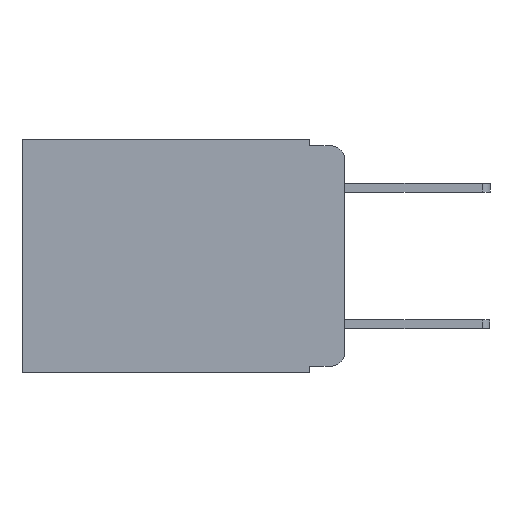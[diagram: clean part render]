
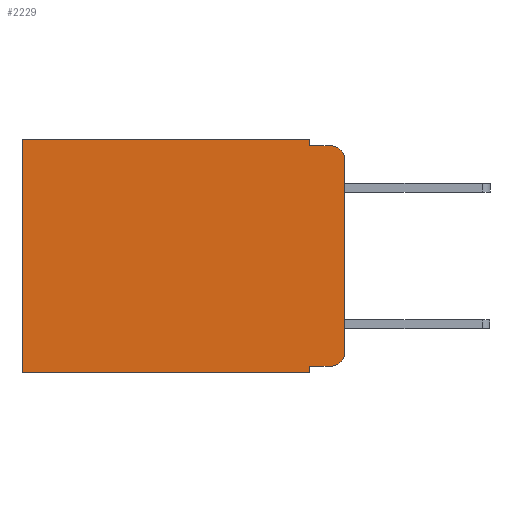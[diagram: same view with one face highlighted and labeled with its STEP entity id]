
A CAD part, left-side view. The second image highlights one B-rep face of the part: STEP entity #2229.
In plain terms, the highlighted planar face has unit normal (-1, 0, 0).
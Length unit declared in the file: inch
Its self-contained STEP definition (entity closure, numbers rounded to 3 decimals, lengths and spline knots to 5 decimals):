
#175 = DIRECTION ( 'NONE',  ( 0., 0., -1. ) ) ;
#256 = LINE ( 'NONE', #12003, #15905 ) ;
#1143 = CARTESIAN_POINT ( 'NONE',  ( 0.298, 0.051, 0. ) ) ;
#1235 = DIRECTION ( 'NONE',  ( 0., 0., -1. ) ) ;
#1457 = CARTESIAN_POINT ( 'NONE',  ( 0.298, 0.051, -0.01 ) ) ;
#2229 = ADVANCED_FACE ( 'NONE', ( #23597 ), #5208, .F. ) ;
#2523 = VECTOR ( 'NONE', #5077, 39.37008 ) ;
#3891 = VERTEX_POINT ( 'NONE', #1457 ) ;
#4057 = CARTESIAN_POINT ( 'NONE',  ( 0.298, 0.473, 0. ) ) ;
#4438 = ORIENTED_EDGE ( 'NONE', *, *, #21599, .F. ) ;
#5017 = ORIENTED_EDGE ( 'NONE', *, *, #8506, .F. ) ;
#5077 = DIRECTION ( 'NONE',  ( 0., 1., 0. ) ) ;
#5208 = PLANE ( 'NONE',  #17487 ) ;
#5235 = ORIENTED_EDGE ( 'NONE', *, *, #22864, .T. ) ;
#6988 = CARTESIAN_POINT ( 'NONE',  ( 0.298, 0., 0. ) ) ;
#7671 = LINE ( 'NONE', #4057, #17326 ) ;
#8372 = VERTEX_POINT ( 'NONE', #12893 ) ;
#8390 = VERTEX_POINT ( 'NONE', #9059 ) ;
#8399 = VECTOR ( 'NONE', #24772, 39.37008 ) ;
#8437 = EDGE_CURVE ( 'NONE', #8372, #10071, #20435, .T. ) ;
#8506 = EDGE_CURVE ( 'NONE', #10071, #21179, #24257, .T. ) ;
#8707 = CARTESIAN_POINT ( 'NONE',  ( 0.298, 0.051, -0.343 ) ) ;
#8765 = EDGE_CURVE ( 'NONE', #13144, #8390, #13245, .T. ) ;
#8959 = EDGE_CURVE ( 'NONE', #24262, #14760, #18016, .T. ) ;
#9059 = CARTESIAN_POINT ( 'NONE',  ( 0.298, 0., -0.313 ) ) ;
#9343 = LINE ( 'NONE', #13038, #18999 ) ;
#9517 = DIRECTION ( 'NONE',  ( -1., 0., 0. ) ) ;
#10071 = VERTEX_POINT ( 'NONE', #8707 ) ;
#10204 = VECTOR ( 'NONE', #13134, 39.37008 ) ;
#11186 = CARTESIAN_POINT ( 'NONE',  ( 0.298, 0.051, 0. ) ) ;
#11949 = CARTESIAN_POINT ( 'NONE',  ( 0.298, 0.473, 0. ) ) ;
#12003 = CARTESIAN_POINT ( 'NONE',  ( 0.298, 0.051, -0.333 ) ) ;
#12038 = CARTESIAN_POINT ( 'NONE',  ( 0.298, 0.051, 0. ) ) ;
#12306 = VERTEX_POINT ( 'NONE', #25038 ) ;
#12382 = ORIENTED_EDGE ( 'NONE', *, *, #8437, .F. ) ;
#12893 = CARTESIAN_POINT ( 'NONE',  ( 0.298, 0.051, -0.333 ) ) ;
#12936 = ORIENTED_EDGE ( 'NONE', *, *, #8959, .T. ) ;
#12988 = DIRECTION ( 'NONE',  ( -1., 0., 0. ) ) ;
#13038 = CARTESIAN_POINT ( 'NONE',  ( 0.298, 0.051, -0.01 ) ) ;
#13134 = DIRECTION ( 'NONE',  ( 0., 0., -1. ) ) ;
#13144 = VERTEX_POINT ( 'NONE', #24255 ) ;
#13245 = LINE ( 'NONE', #21793, #22180 ) ;
#13333 = DIRECTION ( 'NONE',  ( 0., 0., -1. ) ) ;
#13365 = CIRCLE ( 'NONE', #15643, 0.02 ) ;
#13381 = DIRECTION ( 'NONE',  ( 1., 0., 0. ) ) ;
#13408 = CARTESIAN_POINT ( 'NONE',  ( 0.298, 0., 0. ) ) ;
#13617 = ORIENTED_EDGE ( 'NONE', *, *, #18262, .T. ) ;
#14177 = ORIENTED_EDGE ( 'NONE', *, *, #8765, .F. ) ;
#14657 = CARTESIAN_POINT ( 'NONE',  ( 0.298, 0.02, -0.01 ) ) ;
#14760 = VERTEX_POINT ( 'NONE', #11949 ) ;
#15187 = EDGE_CURVE ( 'NONE', #14760, #21179, #7671, .T. ) ;
#15643 = AXIS2_PLACEMENT_3D ( 'NONE', #24374, #12988, #1235 ) ;
#15750 = DIRECTION ( 'NONE',  ( 0., -1., 0. ) ) ;
#15905 = VECTOR ( 'NONE', #15750, 39.37008 ) ;
#16873 = DIRECTION ( 'NONE',  ( 0., -1., 0. ) ) ;
#17142 = CARTESIAN_POINT ( 'NONE',  ( 0.298, 0., -0.343 ) ) ;
#17297 = ORIENTED_EDGE ( 'NONE', *, *, #23046, .T. ) ;
#17326 = VECTOR ( 'NONE', #17578, 39.37008 ) ;
#17487 = AXIS2_PLACEMENT_3D ( 'NONE', #13408, #13381, #13333 ) ;
#17533 = EDGE_LOOP ( 'NONE', ( #14177, #5235, #4438, #21761, #12936, #22007, #5017, #12382, #17297, #13617 ) ) ;
#17578 = DIRECTION ( 'NONE',  ( 0., 0., -1. ) ) ;
#17765 = EDGE_CURVE ( 'NONE', #24262, #3891, #24082, .T. ) ;
#18016 = LINE ( 'NONE', #6988, #2523 ) ;
#18262 = EDGE_CURVE ( 'NONE', #12306, #8390, #13365, .T. ) ;
#18302 = AXIS2_PLACEMENT_3D ( 'NONE', #21046, #9517, #22927 ) ;
#18479 = VECTOR ( 'NONE', #175, 39.37008 ) ;
#18999 = VECTOR ( 'NONE', #16873, 39.37008 ) ;
#19891 = DIRECTION ( 'NONE',  ( 0., 0., -1. ) ) ;
#20435 = LINE ( 'NONE', #11186, #10204 ) ;
#20909 = VERTEX_POINT ( 'NONE', #14657 ) ;
#21046 = CARTESIAN_POINT ( 'NONE',  ( 0.298, 0.02, -0.03 ) ) ;
#21179 = VERTEX_POINT ( 'NONE', #23211 ) ;
#21599 = EDGE_CURVE ( 'NONE', #3891, #20909, #9343, .T. ) ;
#21761 = ORIENTED_EDGE ( 'NONE', *, *, #17765, .F. ) ;
#21793 = CARTESIAN_POINT ( 'NONE',  ( 0.298, 0., 0. ) ) ;
#22007 = ORIENTED_EDGE ( 'NONE', *, *, #15187, .T. ) ;
#22180 = VECTOR ( 'NONE', #19891, 39.37008 ) ;
#22864 = EDGE_CURVE ( 'NONE', #13144, #20909, #24553, .T. ) ;
#22927 = DIRECTION ( 'NONE',  ( 0., 0., -1. ) ) ;
#23046 = EDGE_CURVE ( 'NONE', #8372, #12306, #256, .T. ) ;
#23211 = CARTESIAN_POINT ( 'NONE',  ( 0.298, 0.473, -0.343 ) ) ;
#23597 = FACE_OUTER_BOUND ( 'NONE', #17533, .T. ) ;
#24082 = LINE ( 'NONE', #12038, #18479 ) ;
#24255 = CARTESIAN_POINT ( 'NONE',  ( 0.298, 0., -0.03 ) ) ;
#24257 = LINE ( 'NONE', #17142, #8399 ) ;
#24262 = VERTEX_POINT ( 'NONE', #1143 ) ;
#24374 = CARTESIAN_POINT ( 'NONE',  ( 0.298, 0.02, -0.313 ) ) ;
#24553 = CIRCLE ( 'NONE', #18302, 0.02 ) ;
#24772 = DIRECTION ( 'NONE',  ( 0., 1., 0. ) ) ;
#25038 = CARTESIAN_POINT ( 'NONE',  ( 0.298, 0.02, -0.333 ) ) ;
